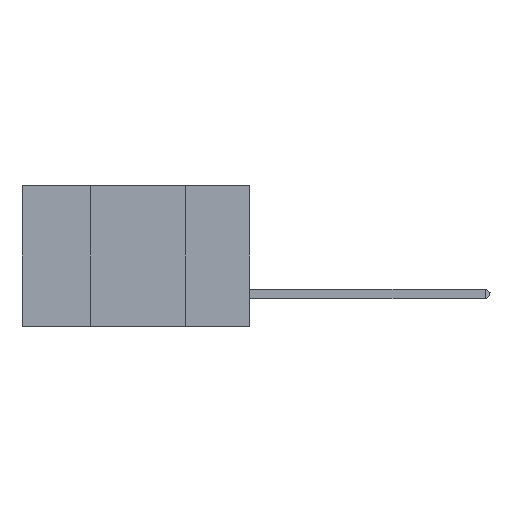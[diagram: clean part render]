
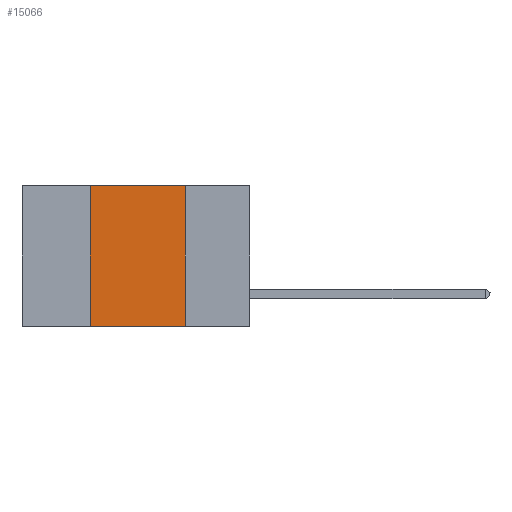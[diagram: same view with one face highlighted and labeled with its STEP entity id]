
A CAD part, left-side view. The second image highlights one B-rep face of the part: STEP entity #15066.
In plain terms, the highlighted planar face has unit normal (-1, 0, 0).
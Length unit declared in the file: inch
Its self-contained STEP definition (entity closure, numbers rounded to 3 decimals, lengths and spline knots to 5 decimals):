
#669 = LINE ( 'NONE', #4614, #12734 ) ;
#1943 = CARTESIAN_POINT ( 'NONE',  ( 0., 0.42, 0. ) ) ;
#2330 = VECTOR ( 'NONE', #32010, 39.37008 ) ;
#4521 = ORIENTED_EDGE ( 'NONE', *, *, #22807, .F. ) ;
#4614 = CARTESIAN_POINT ( 'NONE',  ( 0., 0.6, 0. ) ) ;
#6608 = VERTEX_POINT ( 'NONE', #19880 ) ;
#6890 = VERTEX_POINT ( 'NONE', #38119 ) ;
#7028 = EDGE_LOOP ( 'NONE', ( #21952, #4521, #28284, #19194 ) ) ;
#8070 = VECTOR ( 'NONE', #18046, 39.37008 ) ;
#12734 = VECTOR ( 'NONE', #22938, 39.37008 ) ;
#13736 = VECTOR ( 'NONE', #18156, 39.37008 ) ;
#15066 = ADVANCED_FACE ( 'NONE', ( #32221 ), #28683, .F. ) ;
#16440 = DIRECTION ( 'NONE',  ( 0., 0., -1. ) ) ;
#18033 = CARTESIAN_POINT ( 'NONE',  ( 0., 0.6, -0.37 ) ) ;
#18046 = DIRECTION ( 'NONE',  ( 0., 0., 1. ) ) ;
#18156 = DIRECTION ( 'NONE',  ( 0., -1., 0. ) ) ;
#19194 = ORIENTED_EDGE ( 'NONE', *, *, #20577, .T. ) ;
#19880 = CARTESIAN_POINT ( 'NONE',  ( 0., 0.17, -0.37 ) ) ;
#19976 = VERTEX_POINT ( 'NONE', #1943 ) ;
#20369 = CARTESIAN_POINT ( 'NONE',  ( 0., 0.6, 0. ) ) ;
#20577 = EDGE_CURVE ( 'NONE', #21603, #6608, #29596, .T. ) ;
#21474 = AXIS2_PLACEMENT_3D ( 'NONE', #20369, #34283, #16440 ) ;
#21603 = VERTEX_POINT ( 'NONE', #28102 ) ;
#21952 = ORIENTED_EDGE ( 'NONE', *, *, #32661, .F. ) ;
#22807 = EDGE_CURVE ( 'NONE', #19976, #6890, #669, .T. ) ;
#22938 = DIRECTION ( 'NONE',  ( 0., -1., 0. ) ) ;
#24068 = CARTESIAN_POINT ( 'NONE',  ( 0., 0.42, 0. ) ) ;
#26241 = LINE ( 'NONE', #24068, #8070 ) ;
#28102 = CARTESIAN_POINT ( 'NONE',  ( 0., 0.42, -0.37 ) ) ;
#28284 = ORIENTED_EDGE ( 'NONE', *, *, #30186, .F. ) ;
#28683 = PLANE ( 'NONE',  #21474 ) ;
#29596 = LINE ( 'NONE', #18033, #13736 ) ;
#30186 = EDGE_CURVE ( 'NONE', #21603, #19976, #26241, .T. ) ;
#31637 = LINE ( 'NONE', #35284, #2330 ) ;
#32010 = DIRECTION ( 'NONE',  ( 0., 0., -1. ) ) ;
#32221 = FACE_OUTER_BOUND ( 'NONE', #7028, .T. ) ;
#32661 = EDGE_CURVE ( 'NONE', #6890, #6608, #31637, .T. ) ;
#34283 = DIRECTION ( 'NONE',  ( 1., 0., 0. ) ) ;
#35284 = CARTESIAN_POINT ( 'NONE',  ( 0., 0.17, 0. ) ) ;
#38119 = CARTESIAN_POINT ( 'NONE',  ( 0., 0.17, 0. ) ) ;
